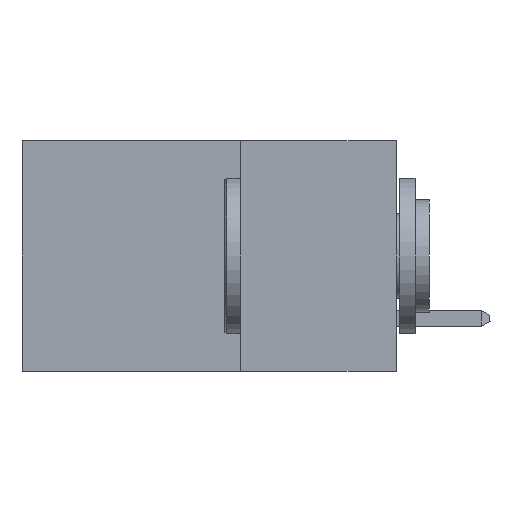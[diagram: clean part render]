
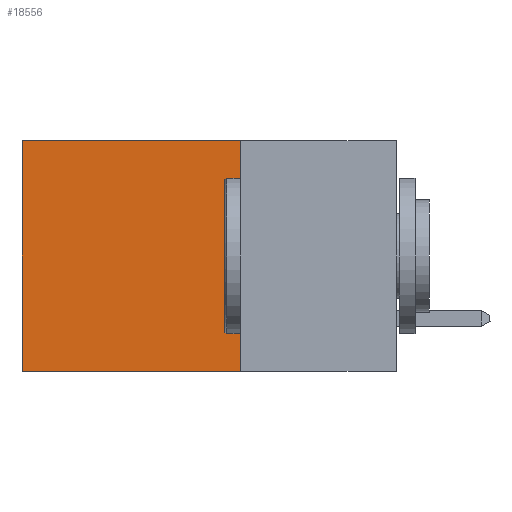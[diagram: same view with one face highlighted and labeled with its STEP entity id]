
A CAD part, left-side view. The second image highlights one B-rep face of the part: STEP entity #18556.
In plain terms, the highlighted planar face has unit normal (-1, 0, 0).
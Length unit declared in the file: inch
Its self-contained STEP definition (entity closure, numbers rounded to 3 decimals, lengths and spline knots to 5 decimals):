
#757 = VERTEX_POINT ( 'NONE', #762 ) ;
#762 = CARTESIAN_POINT ( 'NONE',  ( 0.298, 0.6, -0.37 ) ) ;
#890 = CARTESIAN_POINT ( 'NONE',  ( 0.298, 0.25, 0. ) ) ;
#2682 = CARTESIAN_POINT ( 'NONE',  ( 0.298, 0.25, 0. ) ) ;
#3200 = DIRECTION ( 'NONE',  ( 0., 1., 0. ) ) ;
#4823 = DIRECTION ( 'NONE',  ( 0., 0., -1. ) ) ;
#5049 = ORIENTED_EDGE ( 'NONE', *, *, #15337, .T. ) ;
#5332 = LINE ( 'NONE', #14439, #27329 ) ;
#5352 = CARTESIAN_POINT ( 'NONE',  ( 0.298, 0.25, 0. ) ) ;
#6477 = VECTOR ( 'NONE', #20871, 39.37008 ) ;
#6975 = VERTEX_POINT ( 'NONE', #25353 ) ;
#7226 = VERTEX_POINT ( 'NONE', #890 ) ;
#12398 = ORIENTED_EDGE ( 'NONE', *, *, #23256, .F. ) ;
#13085 = VECTOR ( 'NONE', #22922, 39.37008 ) ;
#13286 = PLANE ( 'NONE',  #18038 ) ;
#13751 = LINE ( 'NONE', #20731, #13085 ) ;
#14439 = CARTESIAN_POINT ( 'NONE',  ( 0.298, 0.6, 0. ) ) ;
#15337 = EDGE_CURVE ( 'NONE', #6975, #757, #5332, .T. ) ;
#15982 = ORIENTED_EDGE ( 'NONE', *, *, #20536, .T. ) ;
#16752 = CARTESIAN_POINT ( 'NONE',  ( 0.298, 0.25, -0.37 ) ) ;
#16773 = EDGE_LOOP ( 'NONE', ( #5049, #12398, #18321, #15982 ) ) ;
#17524 = DIRECTION ( 'NONE',  ( 1., 0., 0. ) ) ;
#18038 = AXIS2_PLACEMENT_3D ( 'NONE', #2682, #17524, #4823 ) ;
#18321 = ORIENTED_EDGE ( 'NONE', *, *, #18905, .F. ) ;
#18556 = ADVANCED_FACE ( 'NONE', ( #26517 ), #13286, .F. ) ;
#18721 = CARTESIAN_POINT ( 'NONE',  ( 0.298, 0.25, 0. ) ) ;
#18905 = EDGE_CURVE ( 'NONE', #7226, #20804, #23506, .T. ) ;
#20536 = EDGE_CURVE ( 'NONE', #7226, #6975, #26592, .T. ) ;
#20731 = CARTESIAN_POINT ( 'NONE',  ( 0.298, 0.25, -0.37 ) ) ;
#20804 = VERTEX_POINT ( 'NONE', #16752 ) ;
#20871 = DIRECTION ( 'NONE',  ( 0., 0., -1. ) ) ;
#20885 = VECTOR ( 'NONE', #3200, 39.37008 ) ;
#22922 = DIRECTION ( 'NONE',  ( 0., 1., 0. ) ) ;
#23256 = EDGE_CURVE ( 'NONE', #20804, #757, #13751, .T. ) ;
#23506 = LINE ( 'NONE', #18721, #6477 ) ;
#25353 = CARTESIAN_POINT ( 'NONE',  ( 0.298, 0.6, 0. ) ) ;
#26517 = FACE_OUTER_BOUND ( 'NONE', #16773, .T. ) ;
#26592 = LINE ( 'NONE', #5352, #20885 ) ;
#27231 = DIRECTION ( 'NONE',  ( 0., 0., -1. ) ) ;
#27329 = VECTOR ( 'NONE', #27231, 39.37008 ) ;
